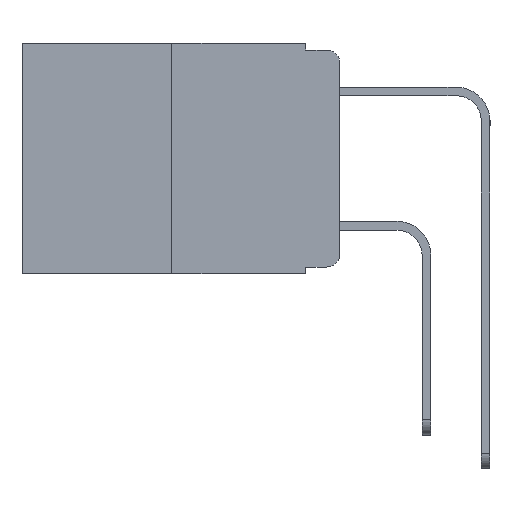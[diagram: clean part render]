
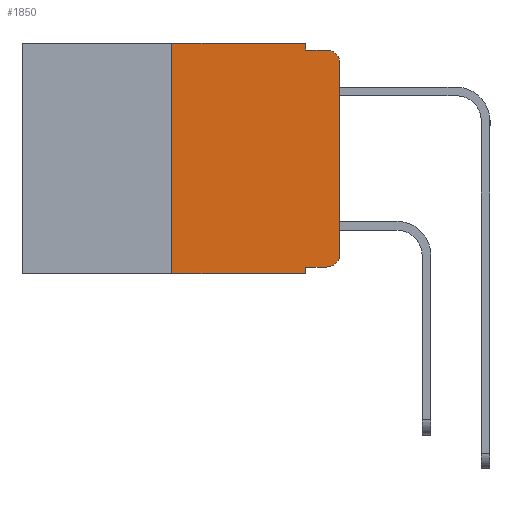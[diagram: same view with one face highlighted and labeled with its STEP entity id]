
A CAD part, left-side view. The second image highlights one B-rep face of the part: STEP entity #1850.
In plain terms, the highlighted planar face has unit normal (-1, 0, 0).
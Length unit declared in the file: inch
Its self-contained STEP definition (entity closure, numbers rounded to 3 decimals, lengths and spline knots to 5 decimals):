
#207 = DIRECTION ( 'NONE',  ( 0., 0., -1. ) ) ;
#375 = VECTOR ( 'NONE', #16009, 39.37008 ) ;
#431 = ORIENTED_EDGE ( 'NONE', *, *, #5007, .T. ) ;
#924 = VERTEX_POINT ( 'NONE', #14429 ) ;
#1222 = LINE ( 'NONE', #5581, #11412 ) ;
#1387 = CARTESIAN_POINT ( 'NONE',  ( 0., 0.25, 0. ) ) ;
#1850 = ADVANCED_FACE ( 'NONE', ( #15484 ), #9494, .F. ) ;
#3141 = ORIENTED_EDGE ( 'NONE', *, *, #21253, .F. ) ;
#3265 = CIRCLE ( 'NONE', #6204, 0.02 ) ;
#3653 = CARTESIAN_POINT ( 'NONE',  ( 0., 0.051, 0. ) ) ;
#4123 = CARTESIAN_POINT ( 'NONE',  ( 0., 0., -0.313 ) ) ;
#4127 = VECTOR ( 'NONE', #21826, 39.37008 ) ;
#4278 = ORIENTED_EDGE ( 'NONE', *, *, #25901, .T. ) ;
#5007 = EDGE_CURVE ( 'NONE', #20789, #6370, #20659, .T. ) ;
#5144 = EDGE_CURVE ( 'NONE', #15202, #924, #22200, .T. ) ;
#5216 = EDGE_CURVE ( 'NONE', #10040, #20789, #10909, .T. ) ;
#5537 = VERTEX_POINT ( 'NONE', #14114 ) ;
#5581 = CARTESIAN_POINT ( 'NONE',  ( 0., 0.473, -0.343 ) ) ;
#6204 = AXIS2_PLACEMENT_3D ( 'NONE', #24405, #12409, #207 ) ;
#6370 = VERTEX_POINT ( 'NONE', #12589 ) ;
#7034 = ORIENTED_EDGE ( 'NONE', *, *, #5216, .T. ) ;
#7042 = ORIENTED_EDGE ( 'NONE', *, *, #5144, .F. ) ;
#7092 = EDGE_CURVE ( 'NONE', #5537, #26101, #20873, .T. ) ;
#7375 = VERTEX_POINT ( 'NONE', #16645 ) ;
#7601 = VECTOR ( 'NONE', #16939, 39.37008 ) ;
#7895 = VERTEX_POINT ( 'NONE', #14324 ) ;
#7982 = CARTESIAN_POINT ( 'NONE',  ( 0., 0., 0. ) ) ;
#9089 = ORIENTED_EDGE ( 'NONE', *, *, #17210, .T. ) ;
#9494 = PLANE ( 'NONE',  #13472 ) ;
#9592 = DIRECTION ( 'NONE',  ( 0., 0., 1. ) ) ;
#10040 = VERTEX_POINT ( 'NONE', #22120 ) ;
#10334 = EDGE_CURVE ( 'NONE', #924, #7375, #23647, .T. ) ;
#10666 = VECTOR ( 'NONE', #9592, 39.37008 ) ;
#10718 = DIRECTION ( 'NONE',  ( -1., 0., 0. ) ) ;
#10909 = CIRCLE ( 'NONE', #25910, 0.02 ) ;
#11133 = VECTOR ( 'NONE', #11751, 39.37008 ) ;
#11303 = LINE ( 'NONE', #1387, #10666 ) ;
#11412 = VECTOR ( 'NONE', #17696, 39.37008 ) ;
#11515 = DIRECTION ( 'NONE',  ( 0., 0., -1. ) ) ;
#11751 = DIRECTION ( 'NONE',  ( 0., -1., 0. ) ) ;
#12409 = DIRECTION ( 'NONE',  ( -1., 0., 0. ) ) ;
#12589 = CARTESIAN_POINT ( 'NONE',  ( 0., 0., -0.03 ) ) ;
#12794 = CARTESIAN_POINT ( 'NONE',  ( 0., 0.25, -0.343 ) ) ;
#13472 = AXIS2_PLACEMENT_3D ( 'NONE', #15454, #23505, #11515 ) ;
#13904 = CARTESIAN_POINT ( 'NONE',  ( 0., 0.25, 0. ) ) ;
#14114 = CARTESIAN_POINT ( 'NONE',  ( 0., 0.051, -0.333 ) ) ;
#14324 = CARTESIAN_POINT ( 'NONE',  ( 0., 0.02, -0.01 ) ) ;
#14429 = CARTESIAN_POINT ( 'NONE',  ( 0., 0.051, 0. ) ) ;
#14495 = CARTESIAN_POINT ( 'NONE',  ( 0., 0.051, -0.343 ) ) ;
#14836 = EDGE_LOOP ( 'NONE', ( #431, #9089, #3141, #20788, #7042, #25665, #16533, #16013, #4278, #7034 ) ) ;
#15202 = VERTEX_POINT ( 'NONE', #13904 ) ;
#15303 = VECTOR ( 'NONE', #26004, 39.37008 ) ;
#15454 = CARTESIAN_POINT ( 'NONE',  ( 0., 0.473, 0. ) ) ;
#15484 = FACE_OUTER_BOUND ( 'NONE', #14836, .T. ) ;
#15710 = EDGE_CURVE ( 'NONE', #16133, #15202, #11303, .T. ) ;
#16009 = DIRECTION ( 'NONE',  ( 0., -1., 0. ) ) ;
#16013 = ORIENTED_EDGE ( 'NONE', *, *, #7092, .F. ) ;
#16133 = VERTEX_POINT ( 'NONE', #12794 ) ;
#16469 = LINE ( 'NONE', #19755, #11133 ) ;
#16533 = ORIENTED_EDGE ( 'NONE', *, *, #21836, .T. ) ;
#16568 = LINE ( 'NONE', #23979, #375 ) ;
#16645 = CARTESIAN_POINT ( 'NONE',  ( 0., 0.051, -0.01 ) ) ;
#16877 = VECTOR ( 'NONE', #22475, 39.37008 ) ;
#16939 = DIRECTION ( 'NONE',  ( 0., 0., -1. ) ) ;
#17210 = EDGE_CURVE ( 'NONE', #6370, #7895, #3265, .T. ) ;
#17696 = DIRECTION ( 'NONE',  ( 0., -1., 0. ) ) ;
#18978 = CARTESIAN_POINT ( 'NONE',  ( 0., 0.051, 0. ) ) ;
#19755 = CARTESIAN_POINT ( 'NONE',  ( 0., 0.051, -0.01 ) ) ;
#20478 = CARTESIAN_POINT ( 'NONE',  ( 0., 0.473, 0. ) ) ;
#20659 = LINE ( 'NONE', #7982, #15303 ) ;
#20788 = ORIENTED_EDGE ( 'NONE', *, *, #10334, .F. ) ;
#20789 = VERTEX_POINT ( 'NONE', #4123 ) ;
#20873 = LINE ( 'NONE', #3653, #4127 ) ;
#21253 = EDGE_CURVE ( 'NONE', #7375, #7895, #16469, .T. ) ;
#21826 = DIRECTION ( 'NONE',  ( 0., 0., -1. ) ) ;
#21836 = EDGE_CURVE ( 'NONE', #16133, #26101, #1222, .T. ) ;
#22120 = CARTESIAN_POINT ( 'NONE',  ( 0., 0.02, -0.333 ) ) ;
#22200 = LINE ( 'NONE', #20478, #16877 ) ;
#22475 = DIRECTION ( 'NONE',  ( 0., -1., 0. ) ) ;
#22739 = CARTESIAN_POINT ( 'NONE',  ( 0., 0.02, -0.313 ) ) ;
#23505 = DIRECTION ( 'NONE',  ( 1., 0., 0. ) ) ;
#23647 = LINE ( 'NONE', #18978, #7601 ) ;
#23979 = CARTESIAN_POINT ( 'NONE',  ( 0., 0.051, -0.333 ) ) ;
#24405 = CARTESIAN_POINT ( 'NONE',  ( 0., 0.02, -0.03 ) ) ;
#24716 = DIRECTION ( 'NONE',  ( 0., 0., -1. ) ) ;
#25665 = ORIENTED_EDGE ( 'NONE', *, *, #15710, .F. ) ;
#25901 = EDGE_CURVE ( 'NONE', #5537, #10040, #16568, .T. ) ;
#25910 = AXIS2_PLACEMENT_3D ( 'NONE', #22739, #10718, #24716 ) ;
#26004 = DIRECTION ( 'NONE',  ( 0., 0., 1. ) ) ;
#26101 = VERTEX_POINT ( 'NONE', #14495 ) ;
